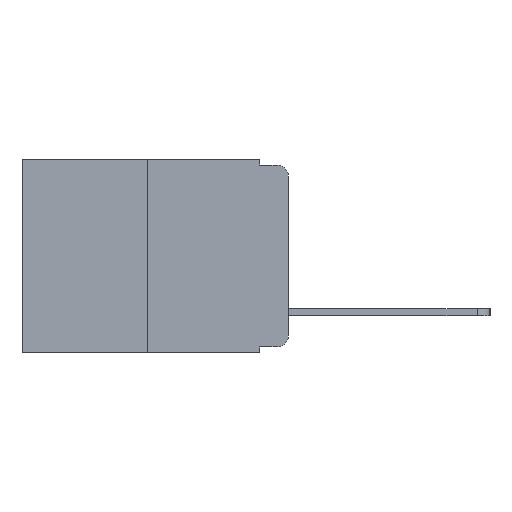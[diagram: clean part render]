
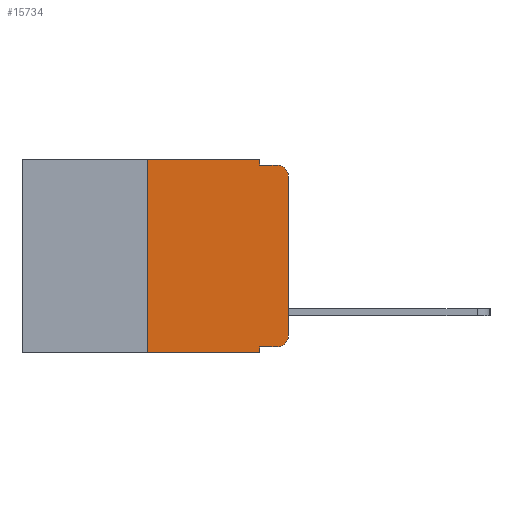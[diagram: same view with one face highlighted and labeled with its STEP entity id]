
A CAD part, left-side view. The second image highlights one B-rep face of the part: STEP entity #15734.
In plain terms, the highlighted planar face has unit normal (-1, 0, 0).
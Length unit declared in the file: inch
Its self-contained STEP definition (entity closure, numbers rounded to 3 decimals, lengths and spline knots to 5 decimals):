
#670 = CIRCLE ( 'NONE', #4049, 0.02 ) ;
#1289 = ORIENTED_EDGE ( 'NONE', *, *, #15636, .F. ) ;
#1349 = LINE ( 'NONE', #6631, #7708 ) ;
#1381 = LINE ( 'NONE', #11580, #4520 ) ;
#1598 = LINE ( 'NONE', #2659, #2011 ) ;
#1650 = EDGE_CURVE ( 'NONE', #15510, #3623, #5499, .T. ) ;
#1712 = VERTEX_POINT ( 'NONE', #4431 ) ;
#1826 = CIRCLE ( 'NONE', #6938, 0.02 ) ;
#2011 = VECTOR ( 'NONE', #12104, 39.37008 ) ;
#2659 = CARTESIAN_POINT ( 'NONE',  ( 0., 0.473, -0.343 ) ) ;
#2957 = ORIENTED_EDGE ( 'NONE', *, *, #9062, .T. ) ;
#2970 = DIRECTION ( 'NONE',  ( 0., 0., 1. ) ) ;
#3070 = FACE_OUTER_BOUND ( 'NONE', #10310, .T. ) ;
#3333 = CARTESIAN_POINT ( 'NONE',  ( 0., 0., -0.03 ) ) ;
#3395 = ORIENTED_EDGE ( 'NONE', *, *, #10274, .T. ) ;
#3407 = VERTEX_POINT ( 'NONE', #13580 ) ;
#3623 = VERTEX_POINT ( 'NONE', #3333 ) ;
#3889 = EDGE_CURVE ( 'NONE', #3407, #15510, #1826, .T. ) ;
#3929 = CARTESIAN_POINT ( 'NONE',  ( 0., 0.473, 0. ) ) ;
#4049 = AXIS2_PLACEMENT_3D ( 'NONE', #14158, #6211, #15401 ) ;
#4431 = CARTESIAN_POINT ( 'NONE',  ( 0., 0.051, 0. ) ) ;
#4520 = VECTOR ( 'NONE', #4842, 39.37008 ) ;
#4568 = VERTEX_POINT ( 'NONE', #12905 ) ;
#4842 = DIRECTION ( 'NONE',  ( 0., 0., -1. ) ) ;
#4889 = VERTEX_POINT ( 'NONE', #9581 ) ;
#5055 = VERTEX_POINT ( 'NONE', #13889 ) ;
#5385 = DIRECTION ( 'NONE',  ( -1., 0., 0. ) ) ;
#5414 = CARTESIAN_POINT ( 'NONE',  ( 0., 0.25, 0. ) ) ;
#5499 = LINE ( 'NONE', #13682, #15211 ) ;
#5724 = ORIENTED_EDGE ( 'NONE', *, *, #15300, .F. ) ;
#6204 = CARTESIAN_POINT ( 'NONE',  ( 0., 0.25, 0. ) ) ;
#6211 = DIRECTION ( 'NONE',  ( -1., 0., 0. ) ) ;
#6593 = ORIENTED_EDGE ( 'NONE', *, *, #16274, .F. ) ;
#6631 = CARTESIAN_POINT ( 'NONE',  ( 0., 0.051, -0.333 ) ) ;
#6880 = CARTESIAN_POINT ( 'NONE',  ( 0., 0.051, -0.333 ) ) ;
#6938 = AXIS2_PLACEMENT_3D ( 'NONE', #13388, #5385, #14663 ) ;
#7020 = ORIENTED_EDGE ( 'NONE', *, *, #3889, .T. ) ;
#7068 = VERTEX_POINT ( 'NONE', #15468 ) ;
#7339 = LINE ( 'NONE', #3929, #10091 ) ;
#7678 = PLANE ( 'NONE',  #9699 ) ;
#7680 = DIRECTION ( 'NONE',  ( 0., 0., -1. ) ) ;
#7708 = VECTOR ( 'NONE', #17093, 39.37008 ) ;
#8119 = EDGE_CURVE ( 'NONE', #4889, #12221, #9466, .T. ) ;
#8470 = CARTESIAN_POINT ( 'NONE',  ( 0., 0.051, 0. ) ) ;
#8502 = ORIENTED_EDGE ( 'NONE', *, *, #10498, .F. ) ;
#8599 = LINE ( 'NONE', #14070, #11308 ) ;
#9062 = EDGE_CURVE ( 'NONE', #4889, #4568, #1598, .T. ) ;
#9466 = LINE ( 'NONE', #6204, #12530 ) ;
#9581 = CARTESIAN_POINT ( 'NONE',  ( 0., 0.25, -0.343 ) ) ;
#9699 = AXIS2_PLACEMENT_3D ( 'NONE', #13953, #15481, #7680 ) ;
#10091 = VECTOR ( 'NONE', #10751, 39.37008 ) ;
#10274 = EDGE_CURVE ( 'NONE', #13048, #3407, #1349, .T. ) ;
#10310 = EDGE_LOOP ( 'NONE', ( #11212, #11629, #1289, #8502, #5724, #16618, #2957, #6593, #3395, #7020 ) ) ;
#10498 = EDGE_CURVE ( 'NONE', #1712, #7068, #15257, .T. ) ;
#10751 = DIRECTION ( 'NONE',  ( 0., -1., 0. ) ) ;
#11200 = CARTESIAN_POINT ( 'NONE',  ( 0., 0., -0.313 ) ) ;
#11212 = ORIENTED_EDGE ( 'NONE', *, *, #1650, .T. ) ;
#11308 = VECTOR ( 'NONE', #15325, 39.37008 ) ;
#11473 = VECTOR ( 'NONE', #13750, 39.37008 ) ;
#11580 = CARTESIAN_POINT ( 'NONE',  ( 0., 0.051, 0. ) ) ;
#11629 = ORIENTED_EDGE ( 'NONE', *, *, #11928, .T. ) ;
#11928 = EDGE_CURVE ( 'NONE', #3623, #5055, #670, .T. ) ;
#12104 = DIRECTION ( 'NONE',  ( 0., -1., 0. ) ) ;
#12221 = VERTEX_POINT ( 'NONE', #5414 ) ;
#12530 = VECTOR ( 'NONE', #12861, 39.37008 ) ;
#12861 = DIRECTION ( 'NONE',  ( 0., 0., 1. ) ) ;
#12905 = CARTESIAN_POINT ( 'NONE',  ( 0., 0.051, -0.343 ) ) ;
#13048 = VERTEX_POINT ( 'NONE', #6880 ) ;
#13388 = CARTESIAN_POINT ( 'NONE',  ( 0., 0.02, -0.313 ) ) ;
#13580 = CARTESIAN_POINT ( 'NONE',  ( 0., 0.02, -0.333 ) ) ;
#13682 = CARTESIAN_POINT ( 'NONE',  ( 0., 0., 0. ) ) ;
#13750 = DIRECTION ( 'NONE',  ( 0., 0., -1. ) ) ;
#13889 = CARTESIAN_POINT ( 'NONE',  ( 0., 0.02, -0.01 ) ) ;
#13953 = CARTESIAN_POINT ( 'NONE',  ( 0., 0.473, 0. ) ) ;
#14070 = CARTESIAN_POINT ( 'NONE',  ( 0., 0.051, -0.01 ) ) ;
#14158 = CARTESIAN_POINT ( 'NONE',  ( 0., 0.02, -0.03 ) ) ;
#14663 = DIRECTION ( 'NONE',  ( 0., 0., -1. ) ) ;
#15211 = VECTOR ( 'NONE', #2970, 39.37008 ) ;
#15257 = LINE ( 'NONE', #8470, #11473 ) ;
#15300 = EDGE_CURVE ( 'NONE', #12221, #1712, #7339, .T. ) ;
#15325 = DIRECTION ( 'NONE',  ( 0., -1., 0. ) ) ;
#15401 = DIRECTION ( 'NONE',  ( 0., 0., -1. ) ) ;
#15468 = CARTESIAN_POINT ( 'NONE',  ( 0., 0.051, -0.01 ) ) ;
#15481 = DIRECTION ( 'NONE',  ( 1., 0., 0. ) ) ;
#15510 = VERTEX_POINT ( 'NONE', #11200 ) ;
#15636 = EDGE_CURVE ( 'NONE', #7068, #5055, #8599, .T. ) ;
#15734 = ADVANCED_FACE ( 'NONE', ( #3070 ), #7678, .F. ) ;
#16274 = EDGE_CURVE ( 'NONE', #13048, #4568, #1381, .T. ) ;
#16618 = ORIENTED_EDGE ( 'NONE', *, *, #8119, .F. ) ;
#17093 = DIRECTION ( 'NONE',  ( 0., -1., 0. ) ) ;
